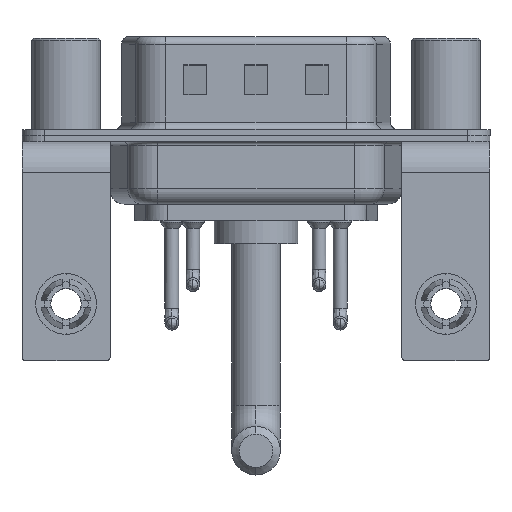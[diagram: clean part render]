
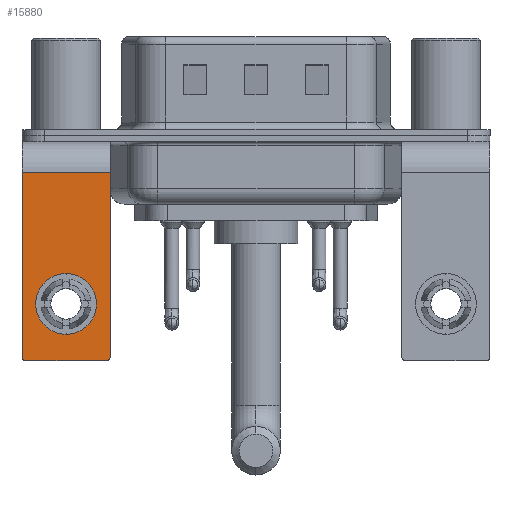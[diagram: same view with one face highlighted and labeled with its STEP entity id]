
A CAD part, front view. The second image highlights one B-rep face of the part: STEP entity #15880.
In plain terms, the highlighted planar face has unit normal (0, -1, 0).
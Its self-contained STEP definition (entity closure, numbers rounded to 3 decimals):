
#44 = DIRECTION ( 'NONE',  ( -1., 0., 0. ) ) ;
#182 = CARTESIAN_POINT ( 'NONE',  ( 0., -6.25, -9.07 ) ) ;
#479 = VECTOR ( 'NONE', #1396, 1000. ) ;
#711 = ORIENTED_EDGE ( 'NONE', *, *, #4374, .F. ) ;
#892 = VERTEX_POINT ( 'NONE', #15152 ) ;
#1276 = DIRECTION ( 'NONE',  ( 0., 1., 0. ) ) ;
#1384 = AXIS2_PLACEMENT_3D ( 'NONE', #2894, #19165, #11673 ) ;
#1396 = DIRECTION ( 'NONE',  ( -1., 0., 0. ) ) ;
#1692 = FACE_BOUND ( 'NONE', #15473, .T. ) ;
#1903 = EDGE_CURVE ( 'NONE', #2419, #2755, #3275, .T. ) ;
#2419 = VERTEX_POINT ( 'NONE', #14401 ) ;
#2755 = VERTEX_POINT ( 'NONE', #18151 ) ;
#2894 = CARTESIAN_POINT ( 'NONE',  ( 0., -6.25, -11.07 ) ) ;
#3095 = CIRCLE ( 'NONE', #16765, 0.25 ) ;
#3275 = LINE ( 'NONE', #5175, #11933 ) ;
#3515 = DIRECTION ( 'NONE',  ( 0., 0., -1. ) ) ;
#4374 = EDGE_CURVE ( 'NONE', #17751, #4981, #10298, .T. ) ;
#4981 = VERTEX_POINT ( 'NONE', #12849 ) ;
#5175 = CARTESIAN_POINT ( 'NONE',  ( 2.9, -6.25, -2.4 ) ) ;
#6341 = ORIENTED_EDGE ( 'NONE', *, *, #1903, .F. ) ;
#6910 = EDGE_CURVE ( 'NONE', #11800, #9141, #18747, .T. ) ;
#7138 = DIRECTION ( 'NONE',  ( 0., 1., 0. ) ) ;
#7445 = AXIS2_PLACEMENT_3D ( 'NONE', #15548, #15311, #18993 ) ;
#7631 = AXIS2_PLACEMENT_3D ( 'NONE', #17549, #1276, #22788 ) ;
#8282 = EDGE_CURVE ( 'NONE', #892, #23391, #20724, .T. ) ;
#8923 = ORIENTED_EDGE ( 'NONE', *, *, #17456, .T. ) ;
#9141 = VERTEX_POINT ( 'NONE', #17299 ) ;
#9288 = VECTOR ( 'NONE', #20651, 1000. ) ;
#10298 = LINE ( 'NONE', #15885, #479 ) ;
#10402 = EDGE_CURVE ( 'NONE', #9141, #4981, #12411, .T. ) ;
#11050 = EDGE_CURVE ( 'NONE', #2419, #11800, #23441, .T. ) ;
#11673 = DIRECTION ( 'NONE',  ( 0., 0., 1. ) ) ;
#11800 = VERTEX_POINT ( 'NONE', #12681 ) ;
#11933 = VECTOR ( 'NONE', #3515, 1000. ) ;
#12411 = CIRCLE ( 'NONE', #7445, 0.25 ) ;
#12618 = PLANE ( 'NONE',  #18605 ) ;
#12681 = CARTESIAN_POINT ( 'NONE',  ( -2.9, -6.25, -2.4 ) ) ;
#12849 = CARTESIAN_POINT ( 'NONE',  ( -2.65, -6.25, -14.8 ) ) ;
#13408 = CARTESIAN_POINT ( 'NONE',  ( -2.9, -6.25, -2.4 ) ) ;
#13535 = DIRECTION ( 'NONE',  ( 0., 0., 1. ) ) ;
#14247 = CARTESIAN_POINT ( 'NONE',  ( 2.65, -6.25, -14.8 ) ) ;
#14287 = FACE_OUTER_BOUND ( 'NONE', #14503, .T. ) ;
#14401 = CARTESIAN_POINT ( 'NONE',  ( 2.9, -6.25, -2.4 ) ) ;
#14407 = CARTESIAN_POINT ( 'NONE',  ( 2.9, -6.25, -2.4 ) ) ;
#14503 = EDGE_LOOP ( 'NONE', ( #21356, #21278, #711, #8923, #6341, #16639 ) ) ;
#15152 = CARTESIAN_POINT ( 'NONE',  ( 0., -6.25, -13.07 ) ) ;
#15311 = DIRECTION ( 'NONE',  ( 0., -1., 0. ) ) ;
#15473 = EDGE_LOOP ( 'NONE', ( #21830, #23274 ) ) ;
#15548 = CARTESIAN_POINT ( 'NONE',  ( -2.65, -6.25, -14.55 ) ) ;
#15880 = ADVANCED_FACE ( 'NONE', ( #1692, #14287 ), #12618, .F. ) ;
#15885 = CARTESIAN_POINT ( 'NONE',  ( 2.9, -6.25, -14.8 ) ) ;
#16639 = ORIENTED_EDGE ( 'NONE', *, *, #11050, .T. ) ;
#16765 = AXIS2_PLACEMENT_3D ( 'NONE', #21011, #20892, #13535 ) ;
#17299 = CARTESIAN_POINT ( 'NONE',  ( -2.9, -6.25, -14.55 ) ) ;
#17456 = EDGE_CURVE ( 'NONE', #17751, #2755, #3095, .T. ) ;
#17549 = CARTESIAN_POINT ( 'NONE',  ( 0., -6.25, -11.07 ) ) ;
#17751 = VERTEX_POINT ( 'NONE', #14247 ) ;
#17962 = DIRECTION ( 'NONE',  ( 0., 0., 1. ) ) ;
#17973 = EDGE_CURVE ( 'NONE', #23391, #892, #22467, .T. ) ;
#18151 = CARTESIAN_POINT ( 'NONE',  ( 2.9, -6.25, -14.55 ) ) ;
#18605 = AXIS2_PLACEMENT_3D ( 'NONE', #23430, #7138, #17962 ) ;
#18747 = LINE ( 'NONE', #13408, #9288 ) ;
#18993 = DIRECTION ( 'NONE',  ( 0., 0., 1. ) ) ;
#19165 = DIRECTION ( 'NONE',  ( 0., 1., 0. ) ) ;
#20651 = DIRECTION ( 'NONE',  ( 0., 0., -1. ) ) ;
#20724 = CIRCLE ( 'NONE', #1384, 2. ) ;
#20892 = DIRECTION ( 'NONE',  ( 0., -1., 0. ) ) ;
#21011 = CARTESIAN_POINT ( 'NONE',  ( 2.65, -6.25, -14.55 ) ) ;
#21278 = ORIENTED_EDGE ( 'NONE', *, *, #10402, .T. ) ;
#21356 = ORIENTED_EDGE ( 'NONE', *, *, #6910, .T. ) ;
#21830 = ORIENTED_EDGE ( 'NONE', *, *, #8282, .T. ) ;
#22467 = CIRCLE ( 'NONE', #7631, 2. ) ;
#22788 = DIRECTION ( 'NONE',  ( 0., 0., 1. ) ) ;
#23274 = ORIENTED_EDGE ( 'NONE', *, *, #17973, .T. ) ;
#23391 = VERTEX_POINT ( 'NONE', #182 ) ;
#23430 = CARTESIAN_POINT ( 'NONE',  ( 2.9, -6.25, -2.4 ) ) ;
#23439 = VECTOR ( 'NONE', #44, 1000. ) ;
#23441 = LINE ( 'NONE', #14407, #23439 ) ;
